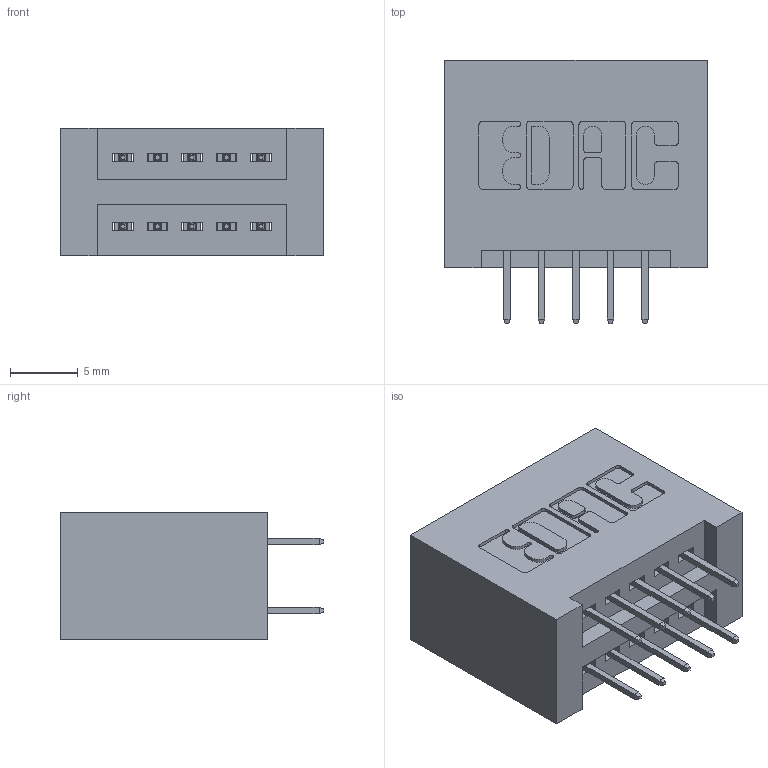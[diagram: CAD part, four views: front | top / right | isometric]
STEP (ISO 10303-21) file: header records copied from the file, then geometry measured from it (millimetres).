
FILE_DESCRIPTION (( 'STEP AP203' ), '1' );
FILE_NAME ('395-010-524-201.STEP', '2018-10-24T04:23:37', ( '' ), ( '' ), 'SwSTEP 2.0', 'SolidWorks 2016', '' );
FILE_SCHEMA (( 'CONFIG_CONTROL_DESIGN' ));
Length unit declared in the file: inch
Products named in the file (3): 345-292-001_345-293-124; 395-010-524-201; 345 Part_No Mounting Lugs
Assembly tree (11 placements, depth 2):
  395-010-524-201
    345 Part_No Mounting Lugs
    345-292-001_345-293-124  x10
Bounding box: 19.3 x 19.35 x 9.4 mm (x, y, z)
Volume: 2132.5 mm3; surface area: 2699 mm2
Topology: 11 solids, 11 shells, 658 faces, 1847 edges, 1190 vertices
Faces by surface type: plane 466, cylinder 192
Entity records: 8701 total; most frequent: CARTESIAN_POINT 1492, ORIENTED_EDGE 1426, DIRECTION 1357, EDGE_CURVE 713, LINE 573, VECTOR 573, VERTEX_POINT 470, AXIS2_PLACEMENT_3D 392
